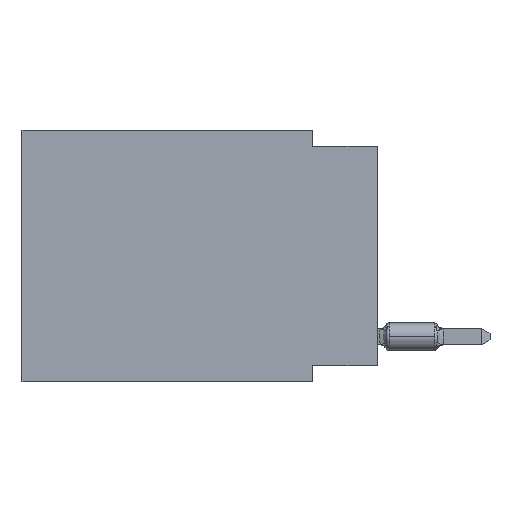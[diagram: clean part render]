
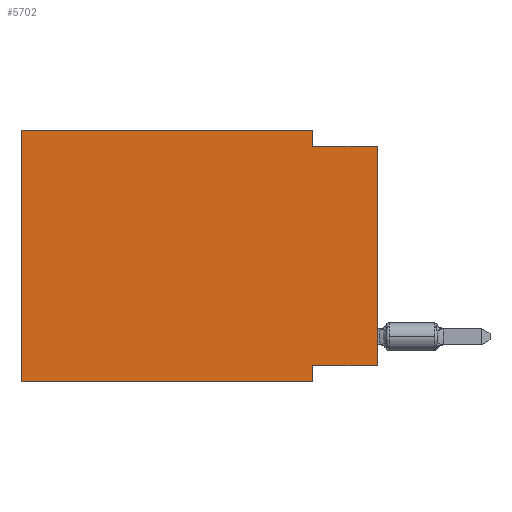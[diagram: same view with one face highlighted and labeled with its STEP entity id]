
A CAD part, left-side view. The second image highlights one B-rep face of the part: STEP entity #5702.
In plain terms, the highlighted planar face has unit normal (-1, 0, 0).
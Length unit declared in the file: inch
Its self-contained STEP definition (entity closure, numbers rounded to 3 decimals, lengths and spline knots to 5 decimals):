
#192 = DIRECTION ( 'NONE',  ( 0., 0., -1. ) ) ;
#234 = ORIENTED_EDGE ( 'NONE', *, *, #13181, .T. ) ;
#468 = VECTOR ( 'NONE', #2666, 39.37008 ) ;
#689 = CARTESIAN_POINT ( 'NONE',  ( 0., 0.1, -0.025 ) ) ;
#1118 = DIRECTION ( 'NONE',  ( 0., -1., 0. ) ) ;
#1377 = LINE ( 'NONE', #15528, #16755 ) ;
#1378 = CARTESIAN_POINT ( 'NONE',  ( 0., 0., 0. ) ) ;
#2460 = EDGE_CURVE ( 'NONE', #11325, #4849, #11356, .T. ) ;
#2468 = EDGE_CURVE ( 'NONE', #2886, #10297, #1377, .T. ) ;
#2666 = DIRECTION ( 'NONE',  ( 0., -1., 0. ) ) ;
#2886 = VERTEX_POINT ( 'NONE', #5529 ) ;
#2936 = FACE_OUTER_BOUND ( 'NONE', #7954, .T. ) ;
#2975 = LINE ( 'NONE', #17394, #6485 ) ;
#3134 = CARTESIAN_POINT ( 'NONE',  ( 0., 0., -0.365 ) ) ;
#3225 = ORIENTED_EDGE ( 'NONE', *, *, #5250, .F. ) ;
#3692 = CARTESIAN_POINT ( 'NONE',  ( 0., 0.55, 0. ) ) ;
#3775 = EDGE_CURVE ( 'NONE', #4849, #6183, #2975, .T. ) ;
#4849 = VERTEX_POINT ( 'NONE', #15465 ) ;
#5101 = AXIS2_PLACEMENT_3D ( 'NONE', #5794, #7372, #12927 ) ;
#5250 = EDGE_CURVE ( 'NONE', #6871, #13031, #5370, .T. ) ;
#5259 = LINE ( 'NONE', #3692, #468 ) ;
#5370 = LINE ( 'NONE', #5555, #5672 ) ;
#5514 = LINE ( 'NONE', #8546, #9493 ) ;
#5529 = CARTESIAN_POINT ( 'NONE',  ( 0., 0.55, -0.39 ) ) ;
#5555 = CARTESIAN_POINT ( 'NONE',  ( 0., 0., -0.025 ) ) ;
#5617 = EDGE_CURVE ( 'NONE', #14114, #6871, #12654, .T. ) ;
#5672 = VECTOR ( 'NONE', #1118, 39.37008 ) ;
#5702 = ADVANCED_FACE ( 'NONE', ( #2936 ), #17067, .F. ) ;
#5794 = CARTESIAN_POINT ( 'NONE',  ( 0., 0.55, 0. ) ) ;
#6183 = VERTEX_POINT ( 'NONE', #10179 ) ;
#6195 = EDGE_CURVE ( 'NONE', #10297, #14114, #5259, .T. ) ;
#6408 = CARTESIAN_POINT ( 'NONE',  ( 0., 0.1, 0. ) ) ;
#6485 = VECTOR ( 'NONE', #192, 39.37008 ) ;
#6871 = VERTEX_POINT ( 'NONE', #689 ) ;
#7372 = DIRECTION ( 'NONE',  ( 1., 0., 0. ) ) ;
#7388 = ORIENTED_EDGE ( 'NONE', *, *, #6195, .F. ) ;
#7788 = CARTESIAN_POINT ( 'NONE',  ( 0., 0., -0.025 ) ) ;
#7954 = EDGE_LOOP ( 'NONE', ( #234, #3225, #8083, #7388, #13123, #13835, #14797, #11707 ) ) ;
#7999 = EDGE_CURVE ( 'NONE', #2886, #6183, #5514, .T. ) ;
#8083 = ORIENTED_EDGE ( 'NONE', *, *, #5617, .F. ) ;
#8534 = CARTESIAN_POINT ( 'NONE',  ( 0., 0., -0.365 ) ) ;
#8546 = CARTESIAN_POINT ( 'NONE',  ( 0., 0.55, -0.39 ) ) ;
#9493 = VECTOR ( 'NONE', #16957, 39.37008 ) ;
#10179 = CARTESIAN_POINT ( 'NONE',  ( 0., 0.1, -0.39 ) ) ;
#10297 = VERTEX_POINT ( 'NONE', #10652 ) ;
#10652 = CARTESIAN_POINT ( 'NONE',  ( 0., 0.55, 0. ) ) ;
#11325 = VERTEX_POINT ( 'NONE', #8534 ) ;
#11356 = LINE ( 'NONE', #3134, #12616 ) ;
#11707 = ORIENTED_EDGE ( 'NONE', *, *, #2460, .F. ) ;
#12389 = CARTESIAN_POINT ( 'NONE',  ( 0., 0.1, 0. ) ) ;
#12616 = VECTOR ( 'NONE', #12852, 39.37008 ) ;
#12654 = LINE ( 'NONE', #12389, #15708 ) ;
#12763 = LINE ( 'NONE', #1378, #17001 ) ;
#12852 = DIRECTION ( 'NONE',  ( 0., 1., 0. ) ) ;
#12927 = DIRECTION ( 'NONE',  ( 0., 0., -1. ) ) ;
#13031 = VERTEX_POINT ( 'NONE', #7788 ) ;
#13123 = ORIENTED_EDGE ( 'NONE', *, *, #2468, .F. ) ;
#13181 = EDGE_CURVE ( 'NONE', #11325, #13031, #12763, .T. ) ;
#13835 = ORIENTED_EDGE ( 'NONE', *, *, #7999, .T. ) ;
#13894 = DIRECTION ( 'NONE',  ( 0., 0., 1. ) ) ;
#13967 = DIRECTION ( 'NONE',  ( 0., 0., -1. ) ) ;
#14114 = VERTEX_POINT ( 'NONE', #6408 ) ;
#14797 = ORIENTED_EDGE ( 'NONE', *, *, #3775, .F. ) ;
#15465 = CARTESIAN_POINT ( 'NONE',  ( 0., 0.1, -0.365 ) ) ;
#15528 = CARTESIAN_POINT ( 'NONE',  ( 0., 0.55, 0. ) ) ;
#15708 = VECTOR ( 'NONE', #13967, 39.37008 ) ;
#16755 = VECTOR ( 'NONE', #16907, 39.37008 ) ;
#16907 = DIRECTION ( 'NONE',  ( 0., 0., 1. ) ) ;
#16957 = DIRECTION ( 'NONE',  ( 0., -1., 0. ) ) ;
#17001 = VECTOR ( 'NONE', #13894, 39.37008 ) ;
#17067 = PLANE ( 'NONE',  #5101 ) ;
#17394 = CARTESIAN_POINT ( 'NONE',  ( 0., 0.1, -0.39 ) ) ;
